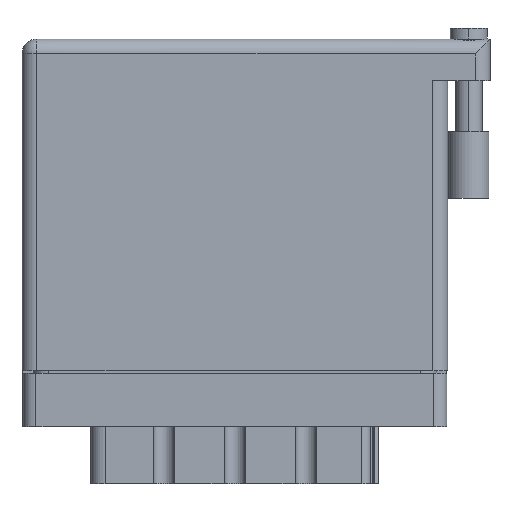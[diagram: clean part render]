
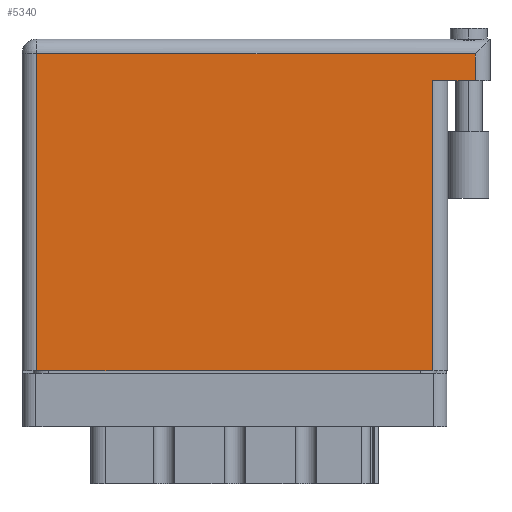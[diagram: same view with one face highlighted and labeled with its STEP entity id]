
A CAD part, front view. The second image highlights one B-rep face of the part: STEP entity #5340.
In plain terms, the highlighted face is planar.
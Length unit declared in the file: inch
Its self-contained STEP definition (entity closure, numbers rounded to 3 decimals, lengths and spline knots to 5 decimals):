
#327 = VERTEX_POINT ( 'NONE', #23040 ) ;
#1753 = EDGE_CURVE ( 'NONE', #11388, #3261, #25862, .T. ) ;
#3219 = CARTESIAN_POINT ( 'NONE',  ( 0., 0., 0. ) ) ;
#3261 = VERTEX_POINT ( 'NONE', #21096 ) ;
#3901 = DIRECTION ( 'NONE',  ( -1., 0., 0. ) ) ;
#5340 = ADVANCED_FACE ( 'NONE', ( #35397 ), #32492, .F. ) ;
#7801 = DIRECTION ( 'NONE',  ( 0., -1., 0. ) ) ;
#8001 = VECTOR ( 'NONE', #34363, 39.37008 ) ;
#8508 = CARTESIAN_POINT ( 'NONE',  ( 0., 1.496, 0. ) ) ;
#9669 = ORIENTED_EDGE ( 'NONE', *, *, #12849, .T. ) ;
#10673 = CARTESIAN_POINT ( 'NONE',  ( 0.07, 1.496, 0. ) ) ;
#11388 = VERTEX_POINT ( 'NONE', #10673 ) ;
#11995 = CARTESIAN_POINT ( 'NONE',  ( 1.938, 1.369, 0. ) ) ;
#12690 = VECTOR ( 'NONE', #17026, 39.37008 ) ;
#12849 = EDGE_CURVE ( 'NONE', #3261, #327, #23195, .T. ) ;
#12994 = LINE ( 'NONE', #15108, #8001 ) ;
#14847 = VECTOR ( 'NONE', #16254, 39.37008 ) ;
#15108 = CARTESIAN_POINT ( 'NONE',  ( 2.138, 1.566, 0. ) ) ;
#15607 = CARTESIAN_POINT ( 'NONE',  ( 2.138, 1.496, 0. ) ) ;
#16029 = EDGE_CURVE ( 'NONE', #21662, #11388, #29165, .T. ) ;
#16254 = DIRECTION ( 'NONE',  ( 1., 0., 0. ) ) ;
#17026 = DIRECTION ( 'NONE',  ( -1., 0., 0. ) ) ;
#18527 = DIRECTION ( 'NONE',  ( -1., 0., 0. ) ) ;
#19112 = ORIENTED_EDGE ( 'NONE', *, *, #1753, .T. ) ;
#20543 = CARTESIAN_POINT ( 'NONE',  ( 0.07, 0., 0. ) ) ;
#20786 = VECTOR ( 'NONE', #18527, 39.37008 ) ;
#20885 = ORIENTED_EDGE ( 'NONE', *, *, #37015, .T. ) ;
#21096 = CARTESIAN_POINT ( 'NONE',  ( 0.07, 0., 0. ) ) ;
#21662 = VERTEX_POINT ( 'NONE', #15607 ) ;
#22753 = VECTOR ( 'NONE', #24417, 39.37008 ) ;
#23040 = CARTESIAN_POINT ( 'NONE',  ( 1.938, 0., 0. ) ) ;
#23195 = LINE ( 'NONE', #3219, #14847 ) ;
#24417 = DIRECTION ( 'NONE',  ( 0., 1., 0. ) ) ;
#25862 = LINE ( 'NONE', #20543, #40192 ) ;
#26122 = VERTEX_POINT ( 'NONE', #33380 ) ;
#26417 = CARTESIAN_POINT ( 'NONE',  ( 0., 1.566, 0. ) ) ;
#26592 = ORIENTED_EDGE ( 'NONE', *, *, #29605, .T. ) ;
#26767 = CARTESIAN_POINT ( 'NONE',  ( 2.208, 1.369, 0. ) ) ;
#26941 = EDGE_CURVE ( 'NONE', #27159, #26122, #36862, .T. ) ;
#27159 = VERTEX_POINT ( 'NONE', #40243 ) ;
#27202 = AXIS2_PLACEMENT_3D ( 'NONE', #26417, #29194, #3901 ) ;
#29165 = LINE ( 'NONE', #8508, #20786 ) ;
#29194 = DIRECTION ( 'NONE',  ( 0., 0., -1. ) ) ;
#29605 = EDGE_CURVE ( 'NONE', #327, #26122, #34103, .T. ) ;
#32492 = PLANE ( 'NONE',  #27202 ) ;
#33380 = CARTESIAN_POINT ( 'NONE',  ( 1.938, 1.369, 0. ) ) ;
#34103 = LINE ( 'NONE', #11995, #22753 ) ;
#34363 = DIRECTION ( 'NONE',  ( 0., 1., 0. ) ) ;
#35397 = FACE_OUTER_BOUND ( 'NONE', #39063, .T. ) ;
#35828 = ORIENTED_EDGE ( 'NONE', *, *, #26941, .F. ) ;
#36862 = LINE ( 'NONE', #26767, #12690 ) ;
#37015 = EDGE_CURVE ( 'NONE', #27159, #21662, #12994, .T. ) ;
#39063 = EDGE_LOOP ( 'NONE', ( #9669, #26592, #35828, #20885, #40854, #19112 ) ) ;
#40192 = VECTOR ( 'NONE', #7801, 39.37008 ) ;
#40243 = CARTESIAN_POINT ( 'NONE',  ( 2.138, 1.369, 0. ) ) ;
#40854 = ORIENTED_EDGE ( 'NONE', *, *, #16029, .T. ) ;
